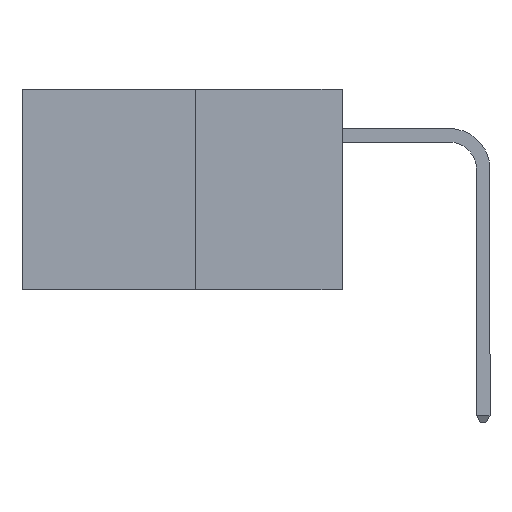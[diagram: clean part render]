
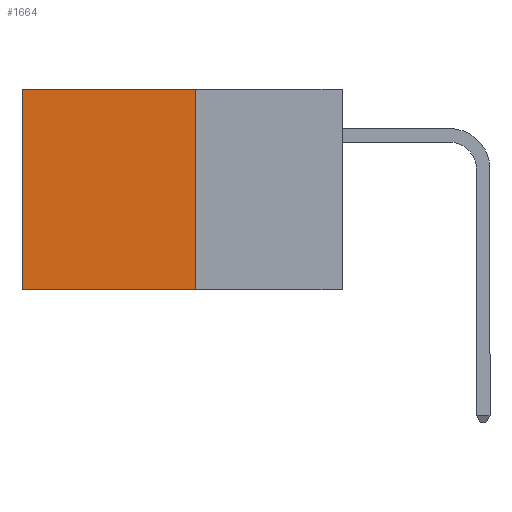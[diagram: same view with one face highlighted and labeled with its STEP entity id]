
A CAD part, left-side view. The second image highlights one B-rep face of the part: STEP entity #1664.
In plain terms, the highlighted planar face has unit normal (-1, 0, 0).
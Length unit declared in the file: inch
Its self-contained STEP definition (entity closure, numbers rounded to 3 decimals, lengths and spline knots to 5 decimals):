
#192 = ORIENTED_EDGE ( 'NONE', *, *, #11925, .F. ) ;
#586 = LINE ( 'NONE', #6122, #5719 ) ;
#801 = EDGE_CURVE ( 'NONE', #10483, #4504, #586, .T. ) ;
#1589 = CARTESIAN_POINT ( 'NONE',  ( 0.277, 0.59, -0.37 ) ) ;
#1608 = VECTOR ( 'NONE', #6615, 39.37008 ) ;
#1664 = ADVANCED_FACE ( 'NONE', ( #10915 ), #6957, .F. ) ;
#2479 = ORIENTED_EDGE ( 'NONE', *, *, #9984, .T. ) ;
#2542 = DIRECTION ( 'NONE',  ( 0., 0., -1. ) ) ;
#2778 = ORIENTED_EDGE ( 'NONE', *, *, #3133, .T. ) ;
#2808 = LINE ( 'NONE', #1589, #9738 ) ;
#3077 = DIRECTION ( 'NONE',  ( 0., 1., 0. ) ) ;
#3133 = EDGE_CURVE ( 'NONE', #4402, #11012, #6700, .T. ) ;
#4402 = VERTEX_POINT ( 'NONE', #8881 ) ;
#4448 = VECTOR ( 'NONE', #10392, 39.37008 ) ;
#4504 = VERTEX_POINT ( 'NONE', #8302 ) ;
#5067 = ORIENTED_EDGE ( 'NONE', *, *, #801, .F. ) ;
#5235 = CARTESIAN_POINT ( 'NONE',  ( 0.277, 0.59, 0. ) ) ;
#5719 = VECTOR ( 'NONE', #3077, 39.37008 ) ;
#6122 = CARTESIAN_POINT ( 'NONE',  ( 0.277, 0.27, -0.37 ) ) ;
#6556 = AXIS2_PLACEMENT_3D ( 'NONE', #7181, #6908, #6902 ) ;
#6563 = CARTESIAN_POINT ( 'NONE',  ( 0.277, 0.27, 0. ) ) ;
#6615 = DIRECTION ( 'NONE',  ( 0., 1., 0. ) ) ;
#6700 = LINE ( 'NONE', #6563, #1608 ) ;
#6902 = DIRECTION ( 'NONE',  ( 0., 0., -1. ) ) ;
#6908 = DIRECTION ( 'NONE',  ( 1., 0., 0. ) ) ;
#6957 = PLANE ( 'NONE',  #6556 ) ;
#6970 = LINE ( 'NONE', #8387, #4448 ) ;
#7181 = CARTESIAN_POINT ( 'NONE',  ( 0.277, 0.27, -0.37 ) ) ;
#8302 = CARTESIAN_POINT ( 'NONE',  ( 0.277, 0.59, -0.37 ) ) ;
#8387 = CARTESIAN_POINT ( 'NONE',  ( 0.277, 0.27, -0.37 ) ) ;
#8881 = CARTESIAN_POINT ( 'NONE',  ( 0.277, 0.27, 0. ) ) ;
#9738 = VECTOR ( 'NONE', #2542, 39.37008 ) ;
#9984 = EDGE_CURVE ( 'NONE', #11012, #4504, #2808, .T. ) ;
#10392 = DIRECTION ( 'NONE',  ( 0., 0., -1. ) ) ;
#10483 = VERTEX_POINT ( 'NONE', #11700 ) ;
#10915 = FACE_OUTER_BOUND ( 'NONE', #12096, .T. ) ;
#11012 = VERTEX_POINT ( 'NONE', #5235 ) ;
#11700 = CARTESIAN_POINT ( 'NONE',  ( 0.277, 0.27, -0.37 ) ) ;
#11925 = EDGE_CURVE ( 'NONE', #4402, #10483, #6970, .T. ) ;
#12096 = EDGE_LOOP ( 'NONE', ( #2479, #5067, #192, #2778 ) ) ;
